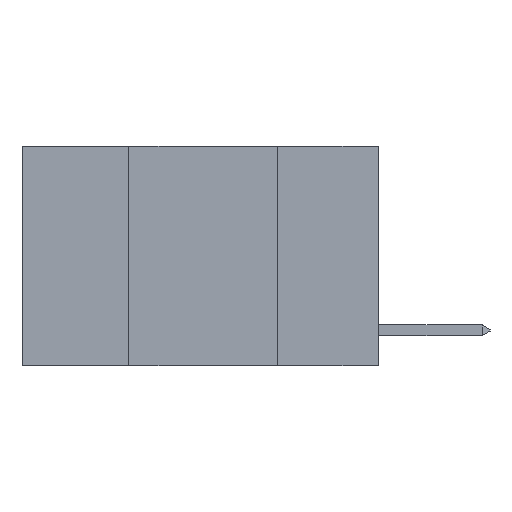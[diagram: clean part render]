
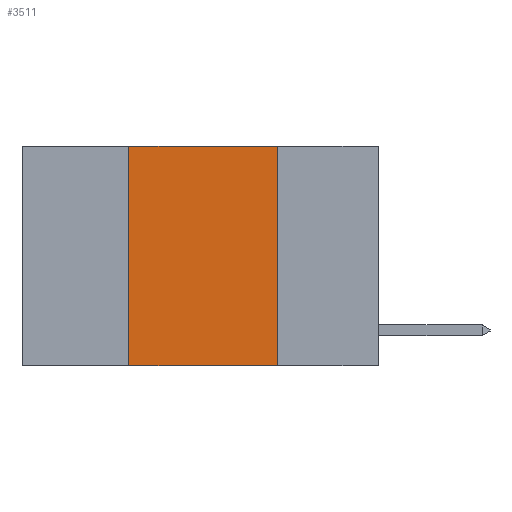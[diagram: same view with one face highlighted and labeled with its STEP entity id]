
A CAD part, left-side view. The second image highlights one B-rep face of the part: STEP entity #3511.
In plain terms, the highlighted planar face has unit normal (-1, 0, 0).
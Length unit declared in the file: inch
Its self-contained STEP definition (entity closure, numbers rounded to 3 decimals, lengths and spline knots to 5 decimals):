
#379 = LINE ( 'NONE', #1390, #4373 ) ;
#472 = CARTESIAN_POINT ( 'NONE',  ( 0., 0.17, 0. ) ) ;
#1002 = EDGE_CURVE ( 'NONE', #8086, #10168, #2686, .T. ) ;
#1191 = EDGE_LOOP ( 'NONE', ( #11490, #11741, #11442, #9004 ) ) ;
#1390 = CARTESIAN_POINT ( 'NONE',  ( 0., 0.6, -0.37 ) ) ;
#1802 = VECTOR ( 'NONE', #3078, 39.37008 ) ;
#1812 = DIRECTION ( 'NONE',  ( 0., 0., -1. ) ) ;
#2294 = DIRECTION ( 'NONE',  ( 0., -1., 0. ) ) ;
#2403 = VECTOR ( 'NONE', #10944, 39.37008 ) ;
#2686 = LINE ( 'NONE', #7461, #2403 ) ;
#2838 = EDGE_CURVE ( 'NONE', #10168, #5108, #9072, .T. ) ;
#3076 = CARTESIAN_POINT ( 'NONE',  ( 0., 0.6, 0. ) ) ;
#3078 = DIRECTION ( 'NONE',  ( 0., -1., 0. ) ) ;
#3499 = VERTEX_POINT ( 'NONE', #6674 ) ;
#3511 = ADVANCED_FACE ( 'NONE', ( #9750 ), #6593, .F. ) ;
#4373 = VECTOR ( 'NONE', #2294, 39.37008 ) ;
#4400 = LINE ( 'NONE', #6329, #9515 ) ;
#5108 = VERTEX_POINT ( 'NONE', #472 ) ;
#6197 = DIRECTION ( 'NONE',  ( 0., 0., -1. ) ) ;
#6236 = DIRECTION ( 'NONE',  ( 1., 0., 0. ) ) ;
#6329 = CARTESIAN_POINT ( 'NONE',  ( 0., 0.17, 0. ) ) ;
#6384 = CARTESIAN_POINT ( 'NONE',  ( 0., 0.6, 0. ) ) ;
#6593 = PLANE ( 'NONE',  #10185 ) ;
#6674 = CARTESIAN_POINT ( 'NONE',  ( 0., 0.17, -0.37 ) ) ;
#7461 = CARTESIAN_POINT ( 'NONE',  ( 0., 0.42, 0. ) ) ;
#7838 = EDGE_CURVE ( 'NONE', #5108, #3499, #4400, .T. ) ;
#8086 = VERTEX_POINT ( 'NONE', #10338 ) ;
#8716 = EDGE_CURVE ( 'NONE', #8086, #3499, #379, .T. ) ;
#9004 = ORIENTED_EDGE ( 'NONE', *, *, #8716, .T. ) ;
#9072 = LINE ( 'NONE', #3076, #1802 ) ;
#9515 = VECTOR ( 'NONE', #1812, 39.37008 ) ;
#9750 = FACE_OUTER_BOUND ( 'NONE', #1191, .T. ) ;
#10168 = VERTEX_POINT ( 'NONE', #10412 ) ;
#10185 = AXIS2_PLACEMENT_3D ( 'NONE', #6384, #6236, #6197 ) ;
#10338 = CARTESIAN_POINT ( 'NONE',  ( 0., 0.42, -0.37 ) ) ;
#10412 = CARTESIAN_POINT ( 'NONE',  ( 0., 0.42, 0. ) ) ;
#10944 = DIRECTION ( 'NONE',  ( 0., 0., 1. ) ) ;
#11442 = ORIENTED_EDGE ( 'NONE', *, *, #1002, .F. ) ;
#11490 = ORIENTED_EDGE ( 'NONE', *, *, #7838, .F. ) ;
#11741 = ORIENTED_EDGE ( 'NONE', *, *, #2838, .F. ) ;
